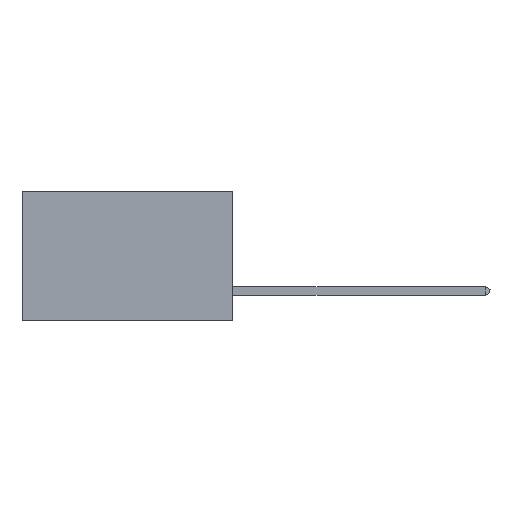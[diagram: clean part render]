
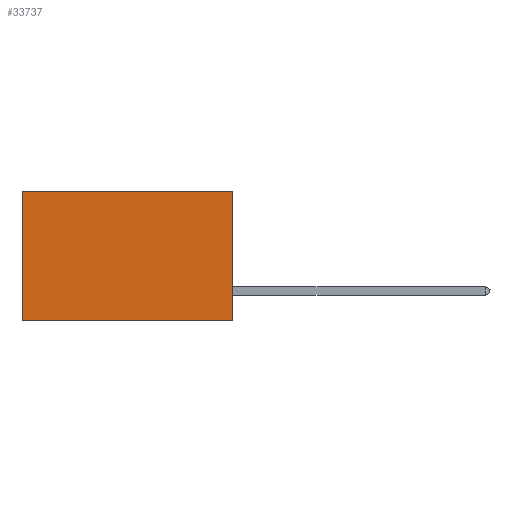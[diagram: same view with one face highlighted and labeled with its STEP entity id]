
A CAD part, left-side view. The second image highlights one B-rep face of the part: STEP entity #33737.
In plain terms, the highlighted planar face has unit normal (-1, 0, 0).
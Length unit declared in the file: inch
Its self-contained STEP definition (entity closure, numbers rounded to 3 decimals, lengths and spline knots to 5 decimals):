
#2804 = PLANE ( 'NONE',  #12254 ) ;
#3195 = ORIENTED_EDGE ( 'NONE', *, *, #12320, .T. ) ;
#4310 = CARTESIAN_POINT ( 'NONE',  ( 0.2875, 0.6, -0.37 ) ) ;
#5434 = FACE_OUTER_BOUND ( 'NONE', #28962, .T. ) ;
#6932 = VECTOR ( 'NONE', #42203, 39.37008 ) ;
#7285 = VECTOR ( 'NONE', #41494, 39.37008 ) ;
#11060 = LINE ( 'NONE', #31426, #37102 ) ;
#11252 = EDGE_CURVE ( 'NONE', #23889, #19970, #11060, .T. ) ;
#12159 = DIRECTION ( 'NONE',  ( 0., 1., 0. ) ) ;
#12254 = AXIS2_PLACEMENT_3D ( 'NONE', #26137, #43059, #19525 ) ;
#12320 = EDGE_CURVE ( 'NONE', #23889, #38092, #24008, .T. ) ;
#14353 = VERTEX_POINT ( 'NONE', #4310 ) ;
#18382 = CARTESIAN_POINT ( 'NONE',  ( 0.2875, 0., 0. ) ) ;
#18762 = VECTOR ( 'NONE', #12159, 39.37008 ) ;
#19525 = DIRECTION ( 'NONE',  ( 0., 0., -1. ) ) ;
#19970 = VERTEX_POINT ( 'NONE', #41573 ) ;
#20452 = ORIENTED_EDGE ( 'NONE', *, *, #11252, .F. ) ;
#23889 = VERTEX_POINT ( 'NONE', #18382 ) ;
#24008 = LINE ( 'NONE', #31948, #7285 ) ;
#24652 = LINE ( 'NONE', #31889, #6932 ) ;
#26137 = CARTESIAN_POINT ( 'NONE',  ( 0.2875, 0., 0. ) ) ;
#27740 = CARTESIAN_POINT ( 'NONE',  ( 0.2875, 0., -0.37 ) ) ;
#28962 = EDGE_LOOP ( 'NONE', ( #42778, #33796, #20452, #3195 ) ) ;
#31426 = CARTESIAN_POINT ( 'NONE',  ( 0.2875, 0., 0. ) ) ;
#31889 = CARTESIAN_POINT ( 'NONE',  ( 0.2875, 0.6, 0. ) ) ;
#31948 = CARTESIAN_POINT ( 'NONE',  ( 0.2875, 0., 0. ) ) ;
#32924 = CARTESIAN_POINT ( 'NONE',  ( 0.2875, 0.6, 0. ) ) ;
#33737 = ADVANCED_FACE ( 'NONE', ( #5434 ), #2804, .F. ) ;
#33796 = ORIENTED_EDGE ( 'NONE', *, *, #36870, .F. ) ;
#34849 = LINE ( 'NONE', #27740, #18762 ) ;
#36870 = EDGE_CURVE ( 'NONE', #19970, #14353, #34849, .T. ) ;
#37102 = VECTOR ( 'NONE', #41317, 39.37008 ) ;
#38092 = VERTEX_POINT ( 'NONE', #32924 ) ;
#40199 = EDGE_CURVE ( 'NONE', #38092, #14353, #24652, .T. ) ;
#41317 = DIRECTION ( 'NONE',  ( 0., 0., -1. ) ) ;
#41494 = DIRECTION ( 'NONE',  ( 0., 1., 0. ) ) ;
#41573 = CARTESIAN_POINT ( 'NONE',  ( 0.2875, 0., -0.37 ) ) ;
#42203 = DIRECTION ( 'NONE',  ( 0., 0., -1. ) ) ;
#42778 = ORIENTED_EDGE ( 'NONE', *, *, #40199, .T. ) ;
#43059 = DIRECTION ( 'NONE',  ( 1., 0., 0. ) ) ;
